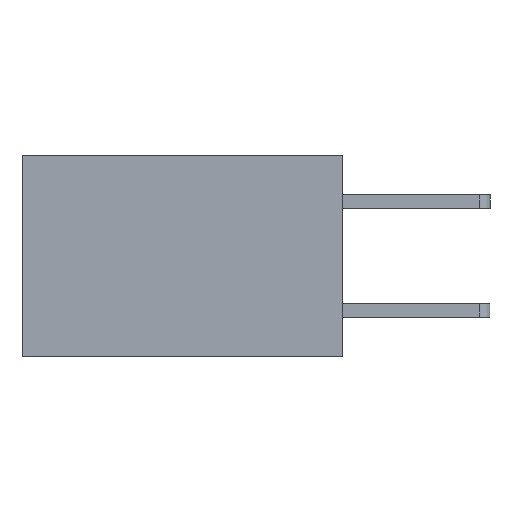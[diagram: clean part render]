
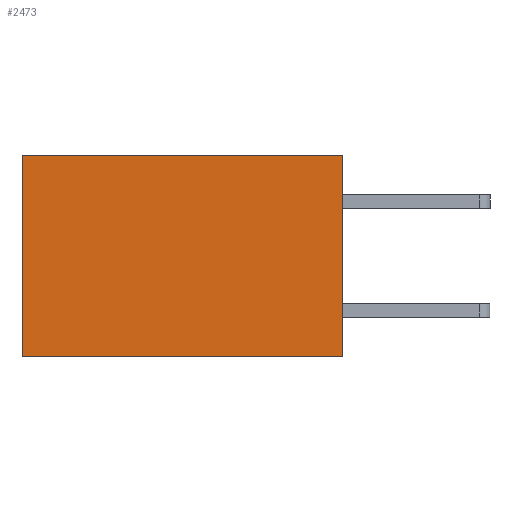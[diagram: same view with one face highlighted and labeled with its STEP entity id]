
A CAD part, left-side view. The second image highlights one B-rep face of the part: STEP entity #2473.
In plain terms, the highlighted planar face has unit normal (-1, 0, 0).
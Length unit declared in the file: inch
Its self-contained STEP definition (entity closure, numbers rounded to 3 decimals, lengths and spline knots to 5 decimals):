
#636 = FACE_OUTER_BOUND ( 'NONE', #2905, .T. ) ;
#729 = CARTESIAN_POINT ( 'NONE',  ( 0.277, 0.59, -0.37 ) ) ;
#797 = EDGE_CURVE ( 'NONE', #2500, #6949, #2911, .T. ) ;
#805 = VECTOR ( 'NONE', #1933, 39.37008 ) ;
#1101 = VERTEX_POINT ( 'NONE', #2115 ) ;
#1184 = EDGE_CURVE ( 'NONE', #4778, #1101, #4825, .T. ) ;
#1696 = CARTESIAN_POINT ( 'NONE',  ( 0.277, 0.59, -0.37 ) ) ;
#1787 = CARTESIAN_POINT ( 'NONE',  ( 0.277, 0., -0.37 ) ) ;
#1933 = DIRECTION ( 'NONE',  ( 0., 1., 0. ) ) ;
#2110 = CARTESIAN_POINT ( 'NONE',  ( 0.277, 0., 0. ) ) ;
#2115 = CARTESIAN_POINT ( 'NONE',  ( 0.277, 0., -0.37 ) ) ;
#2437 = LINE ( 'NONE', #2110, #805 ) ;
#2473 = ADVANCED_FACE ( 'NONE', ( #636 ), #3935, .F. ) ;
#2500 = VERTEX_POINT ( 'NONE', #6717 ) ;
#2895 = DIRECTION ( 'NONE',  ( 0., 0., -1. ) ) ;
#2905 = EDGE_LOOP ( 'NONE', ( #4457, #4571, #4663, #4682 ) ) ;
#2911 = LINE ( 'NONE', #1696, #3852 ) ;
#2946 = VECTOR ( 'NONE', #6153, 39.37008 ) ;
#3655 = EDGE_CURVE ( 'NONE', #1101, #6949, #5814, .T. ) ;
#3852 = VECTOR ( 'NONE', #2895, 39.37008 ) ;
#3935 = PLANE ( 'NONE',  #5602 ) ;
#3968 = DIRECTION ( 'NONE',  ( 0., 0., -1. ) ) ;
#3969 = DIRECTION ( 'NONE',  ( 1., 0., 0. ) ) ;
#4033 = CARTESIAN_POINT ( 'NONE',  ( 0.277, 0., -0.37 ) ) ;
#4457 = ORIENTED_EDGE ( 'NONE', *, *, #797, .T. ) ;
#4571 = ORIENTED_EDGE ( 'NONE', *, *, #3655, .F. ) ;
#4663 = ORIENTED_EDGE ( 'NONE', *, *, #1184, .F. ) ;
#4682 = ORIENTED_EDGE ( 'NONE', *, *, #5894, .T. ) ;
#4778 = VERTEX_POINT ( 'NONE', #5588 ) ;
#4825 = LINE ( 'NONE', #1787, #5943 ) ;
#5064 = DIRECTION ( 'NONE',  ( 0., 0., -1. ) ) ;
#5588 = CARTESIAN_POINT ( 'NONE',  ( 0.277, 0., 0. ) ) ;
#5602 = AXIS2_PLACEMENT_3D ( 'NONE', #4033, #3969, #3968 ) ;
#5814 = LINE ( 'NONE', #6126, #2946 ) ;
#5894 = EDGE_CURVE ( 'NONE', #4778, #2500, #2437, .T. ) ;
#5943 = VECTOR ( 'NONE', #5064, 39.37008 ) ;
#6126 = CARTESIAN_POINT ( 'NONE',  ( 0.277, 0., -0.37 ) ) ;
#6153 = DIRECTION ( 'NONE',  ( 0., 1., 0. ) ) ;
#6717 = CARTESIAN_POINT ( 'NONE',  ( 0.277, 0.59, 0. ) ) ;
#6949 = VERTEX_POINT ( 'NONE', #729 ) ;
